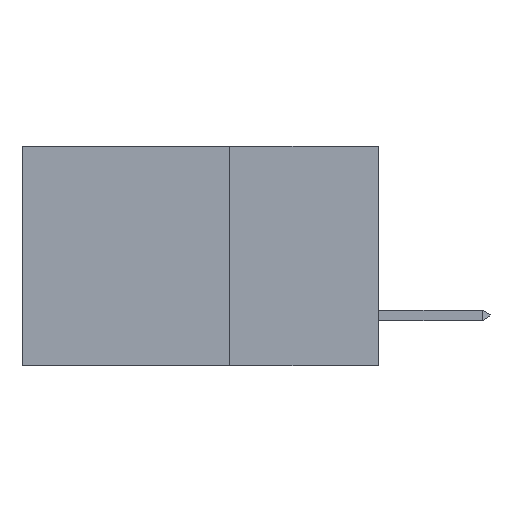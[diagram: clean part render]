
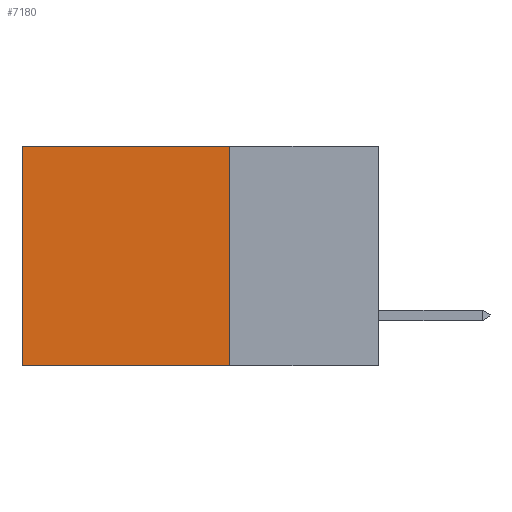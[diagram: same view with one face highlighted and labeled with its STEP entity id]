
A CAD part, left-side view. The second image highlights one B-rep face of the part: STEP entity #7180.
In plain terms, the highlighted planar face has unit normal (-1, 0, 0).
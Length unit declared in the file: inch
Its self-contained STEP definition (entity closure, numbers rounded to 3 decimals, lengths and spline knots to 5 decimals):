
#266 = VERTEX_POINT ( 'NONE', #4304 ) ;
#706 = EDGE_CURVE ( 'NONE', #10137, #5230, #10048, .T. ) ;
#1317 = DIRECTION ( 'NONE',  ( 0., 0., -1. ) ) ;
#1640 = PLANE ( 'NONE',  #12730 ) ;
#2553 = ORIENTED_EDGE ( 'NONE', *, *, #4865, .F. ) ;
#3085 = DIRECTION ( 'NONE',  ( 0., 1., 0. ) ) ;
#3520 = CARTESIAN_POINT ( 'NONE',  ( 0.298, 0.25, 0. ) ) ;
#3522 = CARTESIAN_POINT ( 'NONE',  ( 0.298, 0.25, 0. ) ) ;
#3858 = CARTESIAN_POINT ( 'NONE',  ( 0.298, 0.25, -0.37 ) ) ;
#3934 = DIRECTION ( 'NONE',  ( 0., 0., -1. ) ) ;
#4304 = CARTESIAN_POINT ( 'NONE',  ( 0.298, 0.6, 0. ) ) ;
#4648 = ORIENTED_EDGE ( 'NONE', *, *, #9718, .T. ) ;
#4650 = FACE_OUTER_BOUND ( 'NONE', #13320, .T. ) ;
#4865 = EDGE_CURVE ( 'NONE', #5230, #6924, #7080, .T. ) ;
#5230 = VERTEX_POINT ( 'NONE', #3858 ) ;
#5367 = ORIENTED_EDGE ( 'NONE', *, *, #706, .F. ) ;
#5447 = VECTOR ( 'NONE', #3934, 39.37008 ) ;
#5599 = CARTESIAN_POINT ( 'NONE',  ( 0.298, 0.6, 0. ) ) ;
#5809 = CARTESIAN_POINT ( 'NONE',  ( 0.298, 0.25, 0. ) ) ;
#5889 = CARTESIAN_POINT ( 'NONE',  ( 0.298, 0.25, -0.37 ) ) ;
#6242 = CARTESIAN_POINT ( 'NONE',  ( 0.298, 0.25, 0. ) ) ;
#6374 = VECTOR ( 'NONE', #1317, 39.37008 ) ;
#6793 = DIRECTION ( 'NONE',  ( 0., 0., -1. ) ) ;
#6924 = VERTEX_POINT ( 'NONE', #8076 ) ;
#7080 = LINE ( 'NONE', #5889, #10865 ) ;
#7180 = ADVANCED_FACE ( 'NONE', ( #4650 ), #1640, .F. ) ;
#7308 = LINE ( 'NONE', #3522, #9755 ) ;
#8076 = CARTESIAN_POINT ( 'NONE',  ( 0.298, 0.6, -0.37 ) ) ;
#9718 = EDGE_CURVE ( 'NONE', #266, #6924, #12286, .T. ) ;
#9755 = VECTOR ( 'NONE', #12974, 39.37008 ) ;
#10048 = LINE ( 'NONE', #6242, #5447 ) ;
#10137 = VERTEX_POINT ( 'NONE', #5809 ) ;
#10865 = VECTOR ( 'NONE', #3085, 39.37008 ) ;
#12286 = LINE ( 'NONE', #5599, #6374 ) ;
#12552 = ORIENTED_EDGE ( 'NONE', *, *, #12968, .T. ) ;
#12730 = AXIS2_PLACEMENT_3D ( 'NONE', #3520, #13068, #6793 ) ;
#12968 = EDGE_CURVE ( 'NONE', #10137, #266, #7308, .T. ) ;
#12974 = DIRECTION ( 'NONE',  ( 0., 1., 0. ) ) ;
#13068 = DIRECTION ( 'NONE',  ( 1., 0., 0. ) ) ;
#13320 = EDGE_LOOP ( 'NONE', ( #4648, #2553, #5367, #12552 ) ) ;
